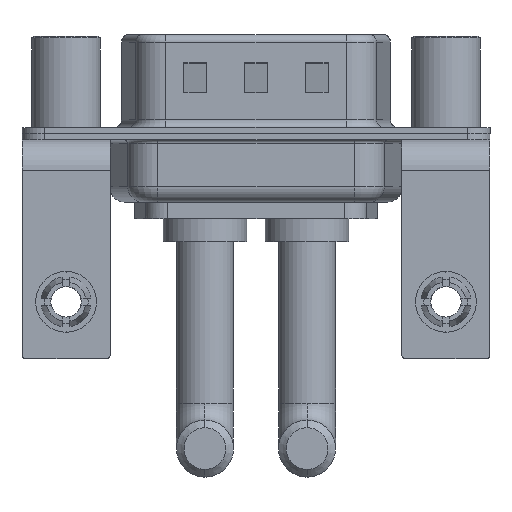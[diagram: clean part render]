
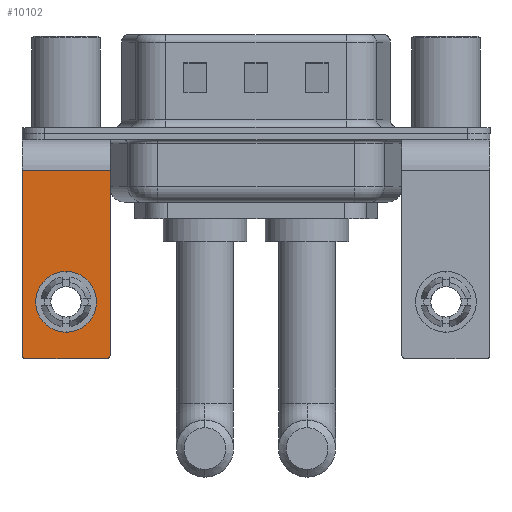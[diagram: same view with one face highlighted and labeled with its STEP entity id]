
A CAD part, front view. The second image highlights one B-rep face of the part: STEP entity #10102.
In plain terms, the highlighted planar face has unit normal (0, -1, 0).
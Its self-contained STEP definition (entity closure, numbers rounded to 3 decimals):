
#47 = DIRECTION ( 'NONE',  ( 0., 0., -1. ) ) ;
#435 = DIRECTION ( 'NONE',  ( -1., 0., 0. ) ) ;
#1035 = DIRECTION ( 'NONE',  ( 0., 0., 1. ) ) ;
#1047 = LINE ( 'NONE', #17434, #2861 ) ;
#1427 = VERTEX_POINT ( 'NONE', #2043 ) ;
#1515 = CIRCLE ( 'NONE', #17132, 2. ) ;
#1706 = CARTESIAN_POINT ( 'NONE',  ( 2.9, -6.25, -2.4 ) ) ;
#1841 = CARTESIAN_POINT ( 'NONE',  ( -2.9, -6.25, -2.4 ) ) ;
#2043 = CARTESIAN_POINT ( 'NONE',  ( 2.9, -6.25, -14.55 ) ) ;
#2361 = ORIENTED_EDGE ( 'NONE', *, *, #17592, .T. ) ;
#2442 = ORIENTED_EDGE ( 'NONE', *, *, #13911, .T. ) ;
#2698 = EDGE_LOOP ( 'NONE', ( #10990, #12858 ) ) ;
#2766 = VECTOR ( 'NONE', #47, 1000. ) ;
#2861 = VECTOR ( 'NONE', #17523, 1000. ) ;
#3430 = DIRECTION ( 'NONE',  ( 0., 1., 0. ) ) ;
#3492 = CARTESIAN_POINT ( 'NONE',  ( 0., -6.25, -9.07 ) ) ;
#4260 = CIRCLE ( 'NONE', #10056, 0.25 ) ;
#4426 = DIRECTION ( 'NONE',  ( 0., -1., 0. ) ) ;
#4704 = CARTESIAN_POINT ( 'NONE',  ( 0., -6.25, -11.07 ) ) ;
#4740 = DIRECTION ( 'NONE',  ( 0., 0., -1. ) ) ;
#4805 = ORIENTED_EDGE ( 'NONE', *, *, #8084, .F. ) ;
#5148 = CIRCLE ( 'NONE', #6291, 0.25 ) ;
#5622 = PLANE ( 'NONE',  #15641 ) ;
#5756 = LINE ( 'NONE', #15510, #2766 ) ;
#5994 = ORIENTED_EDGE ( 'NONE', *, *, #17704, .T. ) ;
#6074 = DIRECTION ( 'NONE',  ( 0., 0., 1. ) ) ;
#6206 = CARTESIAN_POINT ( 'NONE',  ( -2.9, -6.25, -2.4 ) ) ;
#6287 = AXIS2_PLACEMENT_3D ( 'NONE', #12749, #7244, #8692 ) ;
#6291 = AXIS2_PLACEMENT_3D ( 'NONE', #7940, #13427, #1035 ) ;
#6857 = VECTOR ( 'NONE', #4740, 1000. ) ;
#7233 = EDGE_CURVE ( 'NONE', #11692, #1427, #5756, .T. ) ;
#7244 = DIRECTION ( 'NONE',  ( 0., 1., 0. ) ) ;
#7343 = VERTEX_POINT ( 'NONE', #16726 ) ;
#7940 = CARTESIAN_POINT ( 'NONE',  ( -2.65, -6.25, -14.55 ) ) ;
#8084 = EDGE_CURVE ( 'NONE', #17848, #7343, #1047, .T. ) ;
#8547 = VERTEX_POINT ( 'NONE', #13587 ) ;
#8596 = DIRECTION ( 'NONE',  ( 0., 0., 1. ) ) ;
#8601 = DIRECTION ( 'NONE',  ( 0., 0., 1. ) ) ;
#8649 = LINE ( 'NONE', #1841, #6857 ) ;
#8692 = DIRECTION ( 'NONE',  ( 0., 0., 1. ) ) ;
#8783 = FACE_OUTER_BOUND ( 'NONE', #10016, .T. ) ;
#8885 = VECTOR ( 'NONE', #435, 1000. ) ;
#9077 = VERTEX_POINT ( 'NONE', #17396 ) ;
#9342 = CARTESIAN_POINT ( 'NONE',  ( 2.65, -6.25, -14.8 ) ) ;
#9407 = VERTEX_POINT ( 'NONE', #3492 ) ;
#10016 = EDGE_LOOP ( 'NONE', ( #2442, #17293, #4805, #5994, #10089, #2361 ) ) ;
#10056 = AXIS2_PLACEMENT_3D ( 'NONE', #11319, #4426, #8596 ) ;
#10089 = ORIENTED_EDGE ( 'NONE', *, *, #7233, .F. ) ;
#10102 = ADVANCED_FACE ( 'NONE', ( #16827, #8783 ), #5622, .F. ) ;
#10990 = ORIENTED_EDGE ( 'NONE', *, *, #11775, .T. ) ;
#11202 = CIRCLE ( 'NONE', #6287, 2. ) ;
#11319 = CARTESIAN_POINT ( 'NONE',  ( 2.65, -6.25, -14.55 ) ) ;
#11407 = CARTESIAN_POINT ( 'NONE',  ( 2.9, -6.25, -2.4 ) ) ;
#11585 = LINE ( 'NONE', #1706, #8885 ) ;
#11692 = VERTEX_POINT ( 'NONE', #14108 ) ;
#11775 = EDGE_CURVE ( 'NONE', #9077, #9407, #1515, .T. ) ;
#12749 = CARTESIAN_POINT ( 'NONE',  ( 0., -6.25, -11.07 ) ) ;
#12858 = ORIENTED_EDGE ( 'NONE', *, *, #17599, .T. ) ;
#13427 = DIRECTION ( 'NONE',  ( 0., -1., 0. ) ) ;
#13587 = CARTESIAN_POINT ( 'NONE',  ( -2.9, -6.25, -14.55 ) ) ;
#13911 = EDGE_CURVE ( 'NONE', #15204, #8547, #8649, .T. ) ;
#14108 = CARTESIAN_POINT ( 'NONE',  ( 2.9, -6.25, -2.4 ) ) ;
#15204 = VERTEX_POINT ( 'NONE', #6206 ) ;
#15489 = EDGE_CURVE ( 'NONE', #8547, #7343, #5148, .T. ) ;
#15510 = CARTESIAN_POINT ( 'NONE',  ( 2.9, -6.25, -2.4 ) ) ;
#15641 = AXIS2_PLACEMENT_3D ( 'NONE', #11407, #15648, #8601 ) ;
#15648 = DIRECTION ( 'NONE',  ( 0., 1., 0. ) ) ;
#16726 = CARTESIAN_POINT ( 'NONE',  ( -2.65, -6.25, -14.8 ) ) ;
#16827 = FACE_BOUND ( 'NONE', #2698, .T. ) ;
#17132 = AXIS2_PLACEMENT_3D ( 'NONE', #4704, #3430, #6074 ) ;
#17293 = ORIENTED_EDGE ( 'NONE', *, *, #15489, .T. ) ;
#17396 = CARTESIAN_POINT ( 'NONE',  ( 0., -6.25, -13.07 ) ) ;
#17434 = CARTESIAN_POINT ( 'NONE',  ( 2.9, -6.25, -14.8 ) ) ;
#17523 = DIRECTION ( 'NONE',  ( -1., 0., 0. ) ) ;
#17592 = EDGE_CURVE ( 'NONE', #11692, #15204, #11585, .T. ) ;
#17599 = EDGE_CURVE ( 'NONE', #9407, #9077, #11202, .T. ) ;
#17704 = EDGE_CURVE ( 'NONE', #17848, #1427, #4260, .T. ) ;
#17848 = VERTEX_POINT ( 'NONE', #9342 ) ;
